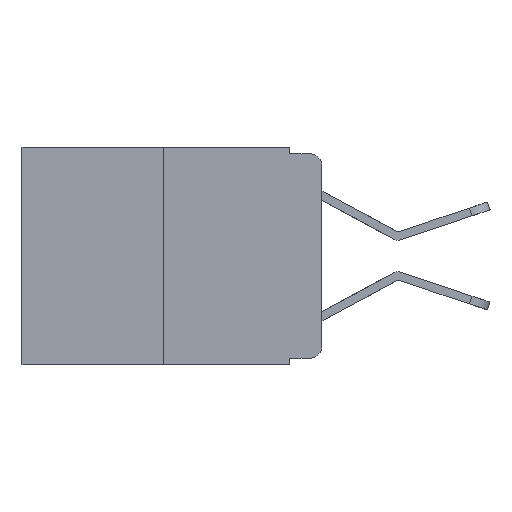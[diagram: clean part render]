
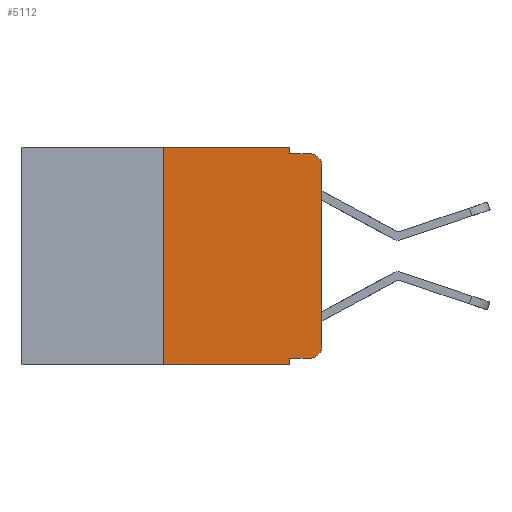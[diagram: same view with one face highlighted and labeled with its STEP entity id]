
A CAD part, left-side view. The second image highlights one B-rep face of the part: STEP entity #5112.
In plain terms, the highlighted planar face has unit normal (-1, 0, 0).
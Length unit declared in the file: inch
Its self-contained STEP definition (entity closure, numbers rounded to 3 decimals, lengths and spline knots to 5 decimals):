
#157 = LINE ( 'NONE', #6561, #10531 ) ;
#603 = CARTESIAN_POINT ( 'NONE',  ( 0., 0., 0. ) ) ;
#864 = VECTOR ( 'NONE', #5399, 39.37008 ) ;
#1332 = VERTEX_POINT ( 'NONE', #8192 ) ;
#1344 = AXIS2_PLACEMENT_3D ( 'NONE', #9808, #4050, #10698 ) ;
#1423 = DIRECTION ( 'NONE',  ( 0., -1., 0. ) ) ;
#1425 = VECTOR ( 'NONE', #11754, 39.37008 ) ;
#1618 = AXIS2_PLACEMENT_3D ( 'NONE', #8884, #2943, #9796 ) ;
#1802 = VERTEX_POINT ( 'NONE', #4111 ) ;
#1852 = ORIENTED_EDGE ( 'NONE', *, *, #9817, .F. ) ;
#1997 = CARTESIAN_POINT ( 'NONE',  ( 0., 0.051, 0. ) ) ;
#2091 = VERTEX_POINT ( 'NONE', #3378 ) ;
#2097 = CARTESIAN_POINT ( 'NONE',  ( 0., 0.051, -0.333 ) ) ;
#2144 = PLANE ( 'NONE',  #10787 ) ;
#2213 = ORIENTED_EDGE ( 'NONE', *, *, #6421, .T. ) ;
#2466 = ORIENTED_EDGE ( 'NONE', *, *, #8597, .F. ) ;
#2943 = DIRECTION ( 'NONE',  ( -1., 0., 0. ) ) ;
#2987 = VERTEX_POINT ( 'NONE', #9984 ) ;
#3134 = DIRECTION ( 'NONE',  ( 0., 0., -1. ) ) ;
#3218 = DIRECTION ( 'NONE',  ( 0., -1., 0. ) ) ;
#3313 = LINE ( 'NONE', #1997, #9874 ) ;
#3368 = EDGE_LOOP ( 'NONE', ( #5036, #2213, #1852, #9552, #11350, #2466, #4413, #4059, #6069, #5132 ) ) ;
#3378 = CARTESIAN_POINT ( 'NONE',  ( 0., 0., -0.313 ) ) ;
#3532 = LINE ( 'NONE', #2097, #5908 ) ;
#3537 = DIRECTION ( 'NONE',  ( 0., -1., 0. ) ) ;
#4013 = VECTOR ( 'NONE', #12372, 39.37008 ) ;
#4050 = DIRECTION ( 'NONE',  ( -1., 0., 0. ) ) ;
#4059 = ORIENTED_EDGE ( 'NONE', *, *, #7990, .F. ) ;
#4111 = CARTESIAN_POINT ( 'NONE',  ( 0., 0.051, -0.333 ) ) ;
#4345 = CARTESIAN_POINT ( 'NONE',  ( 0., 0.25, 0. ) ) ;
#4413 = ORIENTED_EDGE ( 'NONE', *, *, #10344, .T. ) ;
#4662 = CIRCLE ( 'NONE', #1344, 0.02 ) ;
#4963 = VECTOR ( 'NONE', #1423, 39.37008 ) ;
#5036 = ORIENTED_EDGE ( 'NONE', *, *, #7104, .T. ) ;
#5112 = ADVANCED_FACE ( 'NONE', ( #7760 ), #2144, .F. ) ;
#5132 = ORIENTED_EDGE ( 'NONE', *, *, #6660, .T. ) ;
#5399 = DIRECTION ( 'NONE',  ( 0., -1., 0. ) ) ;
#5473 = VERTEX_POINT ( 'NONE', #7571 ) ;
#5579 = CARTESIAN_POINT ( 'NONE',  ( 0., 0.25, -0.343 ) ) ;
#5902 = DIRECTION ( 'NONE',  ( 0., 0., 1. ) ) ;
#5908 = VECTOR ( 'NONE', #3218, 39.37008 ) ;
#6069 = ORIENTED_EDGE ( 'NONE', *, *, #7344, .T. ) ;
#6201 = EDGE_CURVE ( 'NONE', #11849, #5473, #7882, .T. ) ;
#6330 = CARTESIAN_POINT ( 'NONE',  ( 0., 0.473, 0. ) ) ;
#6378 = VECTOR ( 'NONE', #5902, 39.37008 ) ;
#6421 = EDGE_CURVE ( 'NONE', #2987, #10542, #10146, .T. ) ;
#6528 = CARTESIAN_POINT ( 'NONE',  ( 0., 0.051, -0.01 ) ) ;
#6561 = CARTESIAN_POINT ( 'NONE',  ( 0., 0.051, -0.01 ) ) ;
#6660 = EDGE_CURVE ( 'NONE', #9835, #2091, #4662, .T. ) ;
#7104 = EDGE_CURVE ( 'NONE', #2091, #2987, #9706, .T. ) ;
#7335 = DIRECTION ( 'NONE',  ( 0., 0., -1. ) ) ;
#7344 = EDGE_CURVE ( 'NONE', #1802, #9835, #3532, .T. ) ;
#7523 = VERTEX_POINT ( 'NONE', #5579 ) ;
#7571 = CARTESIAN_POINT ( 'NONE',  ( 0., 0.051, 0. ) ) ;
#7599 = CARTESIAN_POINT ( 'NONE',  ( 0., 0.02, -0.01 ) ) ;
#7760 = FACE_OUTER_BOUND ( 'NONE', #3368, .T. ) ;
#7882 = LINE ( 'NONE', #9500, #4963 ) ;
#7990 = EDGE_CURVE ( 'NONE', #1802, #1332, #11554, .T. ) ;
#8192 = CARTESIAN_POINT ( 'NONE',  ( 0., 0.051, -0.343 ) ) ;
#8597 = EDGE_CURVE ( 'NONE', #7523, #11849, #9184, .T. ) ;
#8711 = LINE ( 'NONE', #11895, #864 ) ;
#8884 = CARTESIAN_POINT ( 'NONE',  ( 0., 0.02, -0.03 ) ) ;
#9074 = CARTESIAN_POINT ( 'NONE',  ( 0., 0.051, 0. ) ) ;
#9184 = LINE ( 'NONE', #10659, #4013 ) ;
#9226 = EDGE_CURVE ( 'NONE', #5473, #9464, #3313, .T. ) ;
#9464 = VERTEX_POINT ( 'NONE', #6528 ) ;
#9500 = CARTESIAN_POINT ( 'NONE',  ( 0., 0.473, 0. ) ) ;
#9552 = ORIENTED_EDGE ( 'NONE', *, *, #9226, .F. ) ;
#9706 = LINE ( 'NONE', #603, #6378 ) ;
#9796 = DIRECTION ( 'NONE',  ( 0., 0., -1. ) ) ;
#9808 = CARTESIAN_POINT ( 'NONE',  ( 0., 0.02, -0.313 ) ) ;
#9817 = EDGE_CURVE ( 'NONE', #9464, #10542, #157, .T. ) ;
#9835 = VERTEX_POINT ( 'NONE', #12075 ) ;
#9874 = VECTOR ( 'NONE', #3134, 39.37008 ) ;
#9984 = CARTESIAN_POINT ( 'NONE',  ( 0., 0., -0.03 ) ) ;
#10146 = CIRCLE ( 'NONE', #1618, 0.02 ) ;
#10344 = EDGE_CURVE ( 'NONE', #7523, #1332, #8711, .T. ) ;
#10531 = VECTOR ( 'NONE', #3537, 39.37008 ) ;
#10542 = VERTEX_POINT ( 'NONE', #7599 ) ;
#10659 = CARTESIAN_POINT ( 'NONE',  ( 0., 0.25, 0. ) ) ;
#10698 = DIRECTION ( 'NONE',  ( 0., 0., -1. ) ) ;
#10787 = AXIS2_PLACEMENT_3D ( 'NONE', #6330, #12699, #7335 ) ;
#11350 = ORIENTED_EDGE ( 'NONE', *, *, #6201, .F. ) ;
#11554 = LINE ( 'NONE', #9074, #1425 ) ;
#11754 = DIRECTION ( 'NONE',  ( 0., 0., -1. ) ) ;
#11849 = VERTEX_POINT ( 'NONE', #4345 ) ;
#11895 = CARTESIAN_POINT ( 'NONE',  ( 0., 0.473, -0.343 ) ) ;
#12075 = CARTESIAN_POINT ( 'NONE',  ( 0., 0.02, -0.333 ) ) ;
#12372 = DIRECTION ( 'NONE',  ( 0., 0., 1. ) ) ;
#12699 = DIRECTION ( 'NONE',  ( 1., 0., 0. ) ) ;
